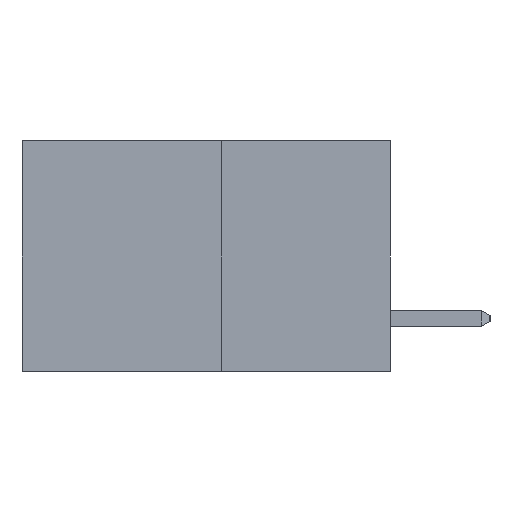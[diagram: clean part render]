
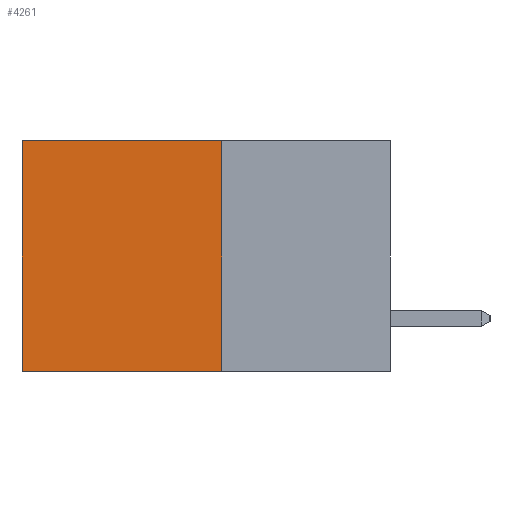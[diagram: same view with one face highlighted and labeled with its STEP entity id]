
A CAD part, left-side view. The second image highlights one B-rep face of the part: STEP entity #4261.
In plain terms, the highlighted planar face has unit normal (-1, 0, 0).
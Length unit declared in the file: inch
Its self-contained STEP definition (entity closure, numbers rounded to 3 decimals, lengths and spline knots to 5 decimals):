
#516 = LINE ( 'NONE', #13224, #19758 ) ;
#692 = CARTESIAN_POINT ( 'NONE',  ( 0.277, 0.59, 0. ) ) ;
#811 = CARTESIAN_POINT ( 'NONE',  ( 0.277, 0.27, 0. ) ) ;
#1806 = CARTESIAN_POINT ( 'NONE',  ( 0.277, 0.27, -0.37 ) ) ;
#2516 = DIRECTION ( 'NONE',  ( 0., 1., 0. ) ) ;
#2928 = CARTESIAN_POINT ( 'NONE',  ( 0.277, 0.59, -0.37 ) ) ;
#2944 = LINE ( 'NONE', #10250, #22649 ) ;
#3601 = DIRECTION ( 'NONE',  ( 0., 0., -1. ) ) ;
#4261 = ADVANCED_FACE ( 'NONE', ( #13790 ), #16422, .F. ) ;
#5661 = VERTEX_POINT ( 'NONE', #811 ) ;
#8284 = DIRECTION ( 'NONE',  ( 0., 0., -1. ) ) ;
#8431 = VERTEX_POINT ( 'NONE', #692 ) ;
#8608 = AXIS2_PLACEMENT_3D ( 'NONE', #16391, #16371, #8284 ) ;
#10250 = CARTESIAN_POINT ( 'NONE',  ( 0.277, 0.27, -0.37 ) ) ;
#11304 = VECTOR ( 'NONE', #21936, 39.37008 ) ;
#11472 = EDGE_CURVE ( 'NONE', #5661, #20302, #516, .T. ) ;
#11765 = EDGE_CURVE ( 'NONE', #20302, #24271, #2944, .T. ) ;
#11986 = LINE ( 'NONE', #12188, #21997 ) ;
#12188 = CARTESIAN_POINT ( 'NONE',  ( 0.277, 0.27, 0. ) ) ;
#13085 = EDGE_CURVE ( 'NONE', #5661, #8431, #11986, .T. ) ;
#13224 = CARTESIAN_POINT ( 'NONE',  ( 0.277, 0.27, -0.37 ) ) ;
#13790 = FACE_OUTER_BOUND ( 'NONE', #17605, .T. ) ;
#14309 = CARTESIAN_POINT ( 'NONE',  ( 0.277, 0.59, -0.37 ) ) ;
#14390 = EDGE_CURVE ( 'NONE', #8431, #24271, #21365, .T. ) ;
#15103 = ORIENTED_EDGE ( 'NONE', *, *, #11472, .F. ) ;
#16371 = DIRECTION ( 'NONE',  ( 1., 0., 0. ) ) ;
#16391 = CARTESIAN_POINT ( 'NONE',  ( 0.277, 0.27, -0.37 ) ) ;
#16422 = PLANE ( 'NONE',  #8608 ) ;
#16979 = ORIENTED_EDGE ( 'NONE', *, *, #11765, .F. ) ;
#17605 = EDGE_LOOP ( 'NONE', ( #18632, #16979, #15103, #17712 ) ) ;
#17712 = ORIENTED_EDGE ( 'NONE', *, *, #13085, .T. ) ;
#18632 = ORIENTED_EDGE ( 'NONE', *, *, #14390, .T. ) ;
#19758 = VECTOR ( 'NONE', #3601, 39.37008 ) ;
#20302 = VERTEX_POINT ( 'NONE', #1806 ) ;
#21365 = LINE ( 'NONE', #14309, #11304 ) ;
#21640 = DIRECTION ( 'NONE',  ( 0., 1., 0. ) ) ;
#21936 = DIRECTION ( 'NONE',  ( 0., 0., -1. ) ) ;
#21997 = VECTOR ( 'NONE', #2516, 39.37008 ) ;
#22649 = VECTOR ( 'NONE', #21640, 39.37008 ) ;
#24271 = VERTEX_POINT ( 'NONE', #2928 ) ;
